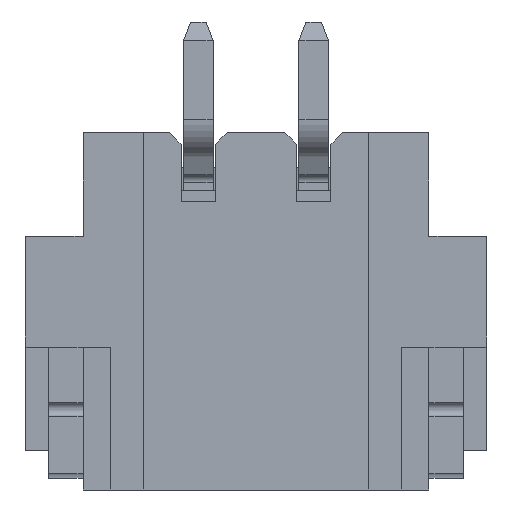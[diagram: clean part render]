
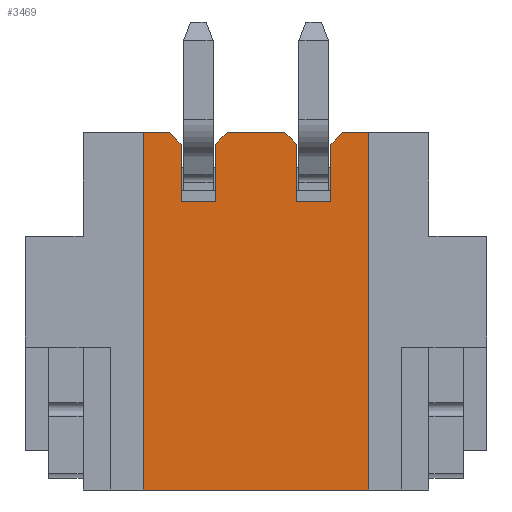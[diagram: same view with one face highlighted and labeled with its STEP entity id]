
A CAD part, front view. The second image highlights one B-rep face of the part: STEP entity #3469.
In plain terms, the highlighted planar face has unit normal (0, -1, 0).
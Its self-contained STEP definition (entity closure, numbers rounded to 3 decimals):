
#109 = DIRECTION ( 'NONE',  ( 1., 0., 0. ) ) ;
#114 = CARTESIAN_POINT ( 'NONE',  ( -2.45, -2.9, -3.875 ) ) ;
#129 = VECTOR ( 'NONE', #1880, 1000. ) ;
#164 = LINE ( 'NONE', #2517, #1814 ) ;
#230 = VERTEX_POINT ( 'NONE', #4723 ) ;
#281 = PLANE ( 'NONE',  #3030 ) ;
#310 = EDGE_CURVE ( 'NONE', #3376, #2776, #4829, .T. ) ;
#393 = EDGE_CURVE ( 'NONE', #3545, #3416, #3347, .T. ) ;
#552 = VERTEX_POINT ( 'NONE', #4124 ) ;
#559 = EDGE_CURVE ( 'NONE', #3193, #4180, #1776, .T. ) ;
#573 = CARTESIAN_POINT ( 'NONE',  ( -1.625, -2.9, 2.375 ) ) ;
#639 = CARTESIAN_POINT ( 'NONE',  ( 0.875, -2.9, 2.375 ) ) ;
#646 = EDGE_CURVE ( 'NONE', #864, #3142, #1323, .T. ) ;
#662 = DIRECTION ( 'NONE',  ( 0., 1., 0. ) ) ;
#683 = VECTOR ( 'NONE', #3414, 1000. ) ;
#698 = ORIENTED_EDGE ( 'NONE', *, *, #3796, .F. ) ;
#760 = LINE ( 'NONE', #1429, #4742 ) ;
#798 = CARTESIAN_POINT ( 'NONE',  ( -1.625, -2.9, 3.625 ) ) ;
#809 = CARTESIAN_POINT ( 'NONE',  ( 1.625, -2.9, 3.625 ) ) ;
#812 = LINE ( 'NONE', #3464, #129 ) ;
#864 = VERTEX_POINT ( 'NONE', #2735 ) ;
#879 = VECTOR ( 'NONE', #1770, 1000. ) ;
#900 = VECTOR ( 'NONE', #1072, 1000. ) ;
#985 = DIRECTION ( 'NONE',  ( -1., 0., 0. ) ) ;
#1021 = CARTESIAN_POINT ( 'NONE',  ( 0.875, -2.9, 2.375 ) ) ;
#1043 = VERTEX_POINT ( 'NONE', #2340 ) ;
#1072 = DIRECTION ( 'NONE',  ( 1., 0., 0. ) ) ;
#1086 = DIRECTION ( 'NONE',  ( 0., 0., 1. ) ) ;
#1109 = CARTESIAN_POINT ( 'NONE',  ( 3.75, -2.9, 3.875 ) ) ;
#1138 = LINE ( 'NONE', #1895, #683 ) ;
#1183 = CARTESIAN_POINT ( 'NONE',  ( -0.625, -2.9, 3.875 ) ) ;
#1298 = CARTESIAN_POINT ( 'NONE',  ( -2.45, -2.9, 3.875 ) ) ;
#1316 = CARTESIAN_POINT ( 'NONE',  ( -0.875, -2.9, 2.375 ) ) ;
#1323 = LINE ( 'NONE', #573, #2515 ) ;
#1347 = CARTESIAN_POINT ( 'NONE',  ( 3.75, -2.9, -3.875 ) ) ;
#1399 = CARTESIAN_POINT ( 'NONE',  ( 2.45, -2.9, 3.875 ) ) ;
#1429 = CARTESIAN_POINT ( 'NONE',  ( -0.875, -2.9, 3.625 ) ) ;
#1518 = EDGE_CURVE ( 'NONE', #1658, #4184, #164, .T. ) ;
#1563 = CARTESIAN_POINT ( 'NONE',  ( 0.875, -2.9, 2.375 ) ) ;
#1587 = ORIENTED_EDGE ( 'NONE', *, *, #2408, .T. ) ;
#1615 = DIRECTION ( 'NONE',  ( -0.707, 0., 0.707 ) ) ;
#1658 = VERTEX_POINT ( 'NONE', #1298 ) ;
#1699 = LINE ( 'NONE', #1347, #2467 ) ;
#1703 = DIRECTION ( 'NONE',  ( 0., 0., -1. ) ) ;
#1728 = DIRECTION ( 'NONE',  ( 0., 0., 1. ) ) ;
#1770 = DIRECTION ( 'NONE',  ( -0.707, 0., -0.707 ) ) ;
#1776 = LINE ( 'NONE', #1399, #3156 ) ;
#1814 = VECTOR ( 'NONE', #1703, 1000. ) ;
#1817 = VECTOR ( 'NONE', #3988, 1000. ) ;
#1818 = EDGE_CURVE ( 'NONE', #3545, #2317, #4172, .T. ) ;
#1847 = CARTESIAN_POINT ( 'NONE',  ( 3.75, -2.9, 3.875 ) ) ;
#1877 = ORIENTED_EDGE ( 'NONE', *, *, #2079, .F. ) ;
#1880 = DIRECTION ( 'NONE',  ( -1., 0., 0. ) ) ;
#1887 = CARTESIAN_POINT ( 'NONE',  ( -0.875, -2.9, 2.375 ) ) ;
#1895 = CARTESIAN_POINT ( 'NONE',  ( 3.75, -2.9, 3.875 ) ) ;
#1921 = CARTESIAN_POINT ( 'NONE',  ( 0.875, -2.9, 3.625 ) ) ;
#1971 = VECTOR ( 'NONE', #2276, 1000. ) ;
#2031 = EDGE_CURVE ( 'NONE', #4180, #4184, #1699, .T. ) ;
#2079 = EDGE_CURVE ( 'NONE', #4716, #1043, #4807, .T. ) ;
#2161 = DIRECTION ( 'NONE',  ( 0., 0., -1. ) ) ;
#2193 = EDGE_CURVE ( 'NONE', #552, #1658, #3711, .T. ) ;
#2276 = DIRECTION ( 'NONE',  ( 0., 0., 1. ) ) ;
#2297 = LINE ( 'NONE', #798, #3584 ) ;
#2317 = VERTEX_POINT ( 'NONE', #2635 ) ;
#2340 = CARTESIAN_POINT ( 'NONE',  ( -0.875, -2.9, 3.625 ) ) ;
#2378 = VERTEX_POINT ( 'NONE', #1183 ) ;
#2381 = ORIENTED_EDGE ( 'NONE', *, *, #310, .T. ) ;
#2408 = EDGE_CURVE ( 'NONE', #3142, #552, #2297, .T. ) ;
#2467 = VECTOR ( 'NONE', #985, 1000. ) ;
#2515 = VECTOR ( 'NONE', #1728, 1000. ) ;
#2517 = CARTESIAN_POINT ( 'NONE',  ( -2.45, -2.9, 3.875 ) ) ;
#2567 = FACE_OUTER_BOUND ( 'NONE', #4713, .T. ) ;
#2615 = VECTOR ( 'NONE', #2627, 1000. ) ;
#2627 = DIRECTION ( 'NONE',  ( 0., 0., 1. ) ) ;
#2635 = CARTESIAN_POINT ( 'NONE',  ( 0.875, -2.9, 3.625 ) ) ;
#2696 = EDGE_CURVE ( 'NONE', #864, #4716, #4633, .T. ) ;
#2735 = CARTESIAN_POINT ( 'NONE',  ( -1.625, -2.9, 2.375 ) ) ;
#2776 = VERTEX_POINT ( 'NONE', #809 ) ;
#2808 = ORIENTED_EDGE ( 'NONE', *, *, #3086, .T. ) ;
#3002 = DIRECTION ( 'NONE',  ( -0.707, 0., -0.707 ) ) ;
#3007 = CARTESIAN_POINT ( 'NONE',  ( -1.625, -2.9, 2.375 ) ) ;
#3030 = AXIS2_PLACEMENT_3D ( 'NONE', #1847, #662, #1086 ) ;
#3086 = EDGE_CURVE ( 'NONE', #2378, #1043, #760, .T. ) ;
#3127 = EDGE_CURVE ( 'NONE', #3193, #3376, #1138, .T. ) ;
#3142 = VERTEX_POINT ( 'NONE', #3457 ) ;
#3156 = VECTOR ( 'NONE', #2161, 1000. ) ;
#3193 = VERTEX_POINT ( 'NONE', #4348 ) ;
#3254 = EDGE_CURVE ( 'NONE', #2317, #230, #4293, .T. ) ;
#3322 = CARTESIAN_POINT ( 'NONE',  ( 1.625, -2.9, 2.375 ) ) ;
#3347 = LINE ( 'NONE', #1563, #3987 ) ;
#3348 = ORIENTED_EDGE ( 'NONE', *, *, #559, .F. ) ;
#3376 = VERTEX_POINT ( 'NONE', #4808 ) ;
#3380 = DIRECTION ( 'NONE',  ( -1., 0., 0. ) ) ;
#3414 = DIRECTION ( 'NONE',  ( -1., 0., 0. ) ) ;
#3416 = VERTEX_POINT ( 'NONE', #4505 ) ;
#3457 = CARTESIAN_POINT ( 'NONE',  ( -1.625, -2.9, 3.625 ) ) ;
#3464 = CARTESIAN_POINT ( 'NONE',  ( 3.75, -2.9, 3.875 ) ) ;
#3469 = ADVANCED_FACE ( 'NONE', ( #2567 ), #281, .F. ) ;
#3482 = ORIENTED_EDGE ( 'NONE', *, *, #3254, .T. ) ;
#3487 = ORIENTED_EDGE ( 'NONE', *, *, #3971, .T. ) ;
#3500 = VECTOR ( 'NONE', #3380, 1000. ) ;
#3531 = ORIENTED_EDGE ( 'NONE', *, *, #2193, .T. ) ;
#3545 = VERTEX_POINT ( 'NONE', #639 ) ;
#3584 = VECTOR ( 'NONE', #3876, 1000. ) ;
#3590 = CARTESIAN_POINT ( 'NONE',  ( 2.45, -2.9, -3.875 ) ) ;
#3620 = ORIENTED_EDGE ( 'NONE', *, *, #646, .T. ) ;
#3711 = LINE ( 'NONE', #1109, #3500 ) ;
#3774 = ORIENTED_EDGE ( 'NONE', *, *, #3127, .T. ) ;
#3796 = EDGE_CURVE ( 'NONE', #3416, #2776, #4159, .T. ) ;
#3876 = DIRECTION ( 'NONE',  ( -0.707, 0., 0.707 ) ) ;
#3971 = EDGE_CURVE ( 'NONE', #230, #2378, #812, .T. ) ;
#3987 = VECTOR ( 'NONE', #109, 1000. ) ;
#3988 = DIRECTION ( 'NONE',  ( 0., 0., 1. ) ) ;
#4124 = CARTESIAN_POINT ( 'NONE',  ( -1.875, -2.9, 3.875 ) ) ;
#4159 = LINE ( 'NONE', #3322, #2615 ) ;
#4172 = LINE ( 'NONE', #1021, #1971 ) ;
#4180 = VERTEX_POINT ( 'NONE', #3590 ) ;
#4184 = VERTEX_POINT ( 'NONE', #114 ) ;
#4293 = LINE ( 'NONE', #1921, #4976 ) ;
#4336 = ORIENTED_EDGE ( 'NONE', *, *, #1818, .T. ) ;
#4348 = CARTESIAN_POINT ( 'NONE',  ( 2.45, -2.9, 3.875 ) ) ;
#4384 = ORIENTED_EDGE ( 'NONE', *, *, #393, .F. ) ;
#4411 = ORIENTED_EDGE ( 'NONE', *, *, #1518, .T. ) ;
#4505 = CARTESIAN_POINT ( 'NONE',  ( 1.625, -2.9, 2.375 ) ) ;
#4524 = CARTESIAN_POINT ( 'NONE',  ( 1.625, -2.9, 3.625 ) ) ;
#4633 = LINE ( 'NONE', #3007, #900 ) ;
#4713 = EDGE_LOOP ( 'NONE', ( #3487, #2808, #1877, #4897, #3620, #1587, #3531, #4411, #4947, #3348, #3774, #2381, #698, #4384, #4336, #3482 ) ) ;
#4716 = VERTEX_POINT ( 'NONE', #1887 ) ;
#4723 = CARTESIAN_POINT ( 'NONE',  ( 0.625, -2.9, 3.875 ) ) ;
#4742 = VECTOR ( 'NONE', #3002, 1000. ) ;
#4807 = LINE ( 'NONE', #1316, #1817 ) ;
#4808 = CARTESIAN_POINT ( 'NONE',  ( 1.875, -2.9, 3.875 ) ) ;
#4829 = LINE ( 'NONE', #4524, #879 ) ;
#4897 = ORIENTED_EDGE ( 'NONE', *, *, #2696, .F. ) ;
#4947 = ORIENTED_EDGE ( 'NONE', *, *, #2031, .F. ) ;
#4976 = VECTOR ( 'NONE', #1615, 1000. ) ;
